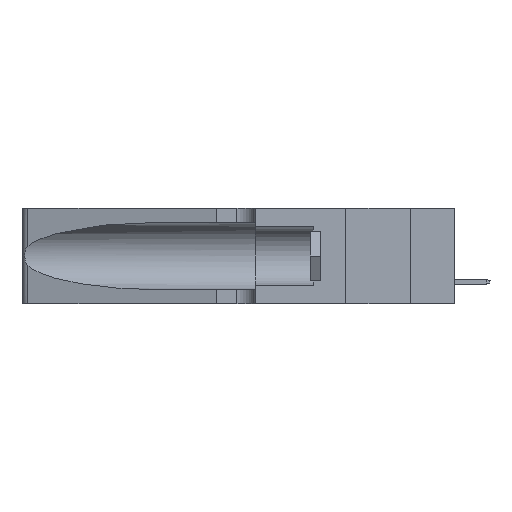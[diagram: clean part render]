
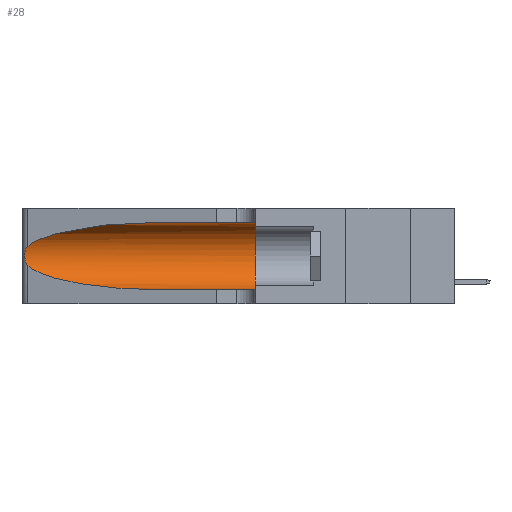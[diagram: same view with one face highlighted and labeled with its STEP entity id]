
A CAD part, left-side view. The second image highlights one B-rep face of the part: STEP entity #28.
In plain terms, the highlighted cylindrical face has radius 3.308 mm (diameter 6.617 mm), a partial arc.
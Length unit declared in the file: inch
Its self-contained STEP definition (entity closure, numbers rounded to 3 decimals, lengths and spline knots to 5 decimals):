
#28 = ADVANCED_FACE ( 'NONE', ( #6190 ), #16689, .F. ) ;
#848 = CARTESIAN_POINT ( 'NONE',  ( 0.25487, 1.22718, 0.14631 ) ) ;
#1458 = EDGE_CURVE ( 'NONE', #31231, #33976, #28889, .T. ) ;
#1917 = VERTEX_POINT ( 'NONE', #17736 ) ;
#2438 = CARTESIAN_POINT ( 'NONE',  ( 0.25487, 1.22718, 0.22369 ) ) ;
#2667 = EDGE_CURVE ( 'NONE', #25643, #31231, #16777, .T. ) ;
#3200 = ORIENTED_EDGE ( 'NONE', *, *, #5541, .F. ) ;
#3679 = CARTESIAN_POINT ( 'NONE',  ( 0.1305, 0.72297, 0.05475 ) ) ;
#3865 = CARTESIAN_POINT ( 'NONE',  ( 0.1305, 0.72297, 0.31525 ) ) ;
#3956 = DIRECTION ( 'NONE',  ( 0., 0., -1. ) ) ;
#4356 = CARTESIAN_POINT ( 'NONE',  ( 0.25487, 1.22718, 0.14631 ) ) ;
#4912 =( BOUNDED_CURVE ( )  B_SPLINE_CURVE ( 3, ( #9679, #20197, #30686, #3679 ),
 .UNSPECIFIED., .F., .T. ) 
 B_SPLINE_CURVE_WITH_KNOTS ( ( 4, 4 ),
 ( 3.44316, 4.71239 ),
 .UNSPECIFIED. ) 
 CURVE ( )  GEOMETRIC_REPRESENTATION_ITEM ( )  RATIONAL_B_SPLINE_CURVE ( ( 1., 0.87, 0.87, 1. ) ) 
 REPRESENTATION_ITEM ( '' )  );
#4992 = DIRECTION ( 'NONE',  ( 0., 1., 0. ) ) ;
#5541 = EDGE_CURVE ( 'NONE', #1917, #24523, #21792, .T. ) ;
#6121 = DIRECTION ( 'NONE',  ( 0., -1., 0. ) ) ;
#6190 = FACE_OUTER_BOUND ( 'NONE', #11603, .T. ) ;
#6216 = VERTEX_POINT ( 'NONE', #15237 ) ;
#6430 = CARTESIAN_POINT ( 'NONE',  ( 0.1305, 1.61858, 0.31525 ) ) ;
#6464 = CARTESIAN_POINT ( 'NONE',  ( 0.1305, 1.61858, 0.05475 ) ) ;
#6635 = EDGE_CURVE ( 'NONE', #33976, #6216, #4912, .T. ) ;
#6663 = EDGE_CURVE ( 'NONE', #25643, #1917, #30012, .T. ) ;
#7116 = ORIENTED_EDGE ( 'NONE', *, *, #6663, .F. ) ;
#7269 = CARTESIAN_POINT ( 'NONE',  ( 0.25639, 1.23186, 0.15144 ) ) ;
#7533 = AXIS2_PLACEMENT_3D ( 'NONE', #27198, #22193, #3956 ) ;
#7562 = VECTOR ( 'NONE', #32745, 39.37008 ) ;
#7593 = CARTESIAN_POINT ( 'NONE',  ( 0.25854, 1.2359, 0.20912 ) ) ;
#7616 = ORIENTED_EDGE ( 'NONE', *, *, #6635, .T. ) ;
#8374 = ORIENTED_EDGE ( 'NONE', *, *, #2667, .T. ) ;
#9072 = CARTESIAN_POINT ( 'NONE',  ( 0.1305, 0.35, 0.05475 ) ) ;
#9679 = CARTESIAN_POINT ( 'NONE',  ( 0.25487, 1.22718, 0.14631 ) ) ;
#10350 = CARTESIAN_POINT ( 'NONE',  ( 0.2373, 1.15595, 0.28018 ) ) ;
#11603 = EDGE_LOOP ( 'NONE', ( #8374, #33777, #7616, #32934, #3200, #7116 ) ) ;
#12437 = CARTESIAN_POINT ( 'NONE',  ( 0.26075, 1.23896, 0.178 ) ) ;
#12606 = CARTESIAN_POINT ( 'NONE',  ( 0.25639, 1.23184, 0.21858 ) ) ;
#15237 = CARTESIAN_POINT ( 'NONE',  ( 0.1305, 0.72297, 0.05475 ) ) ;
#15377 = EDGE_CURVE ( 'NONE', #6216, #24523, #24540, .T. ) ;
#16689 = CYLINDRICAL_SURFACE ( 'NONE', #7533, 0.13025 ) ;
#16777 =( BOUNDED_CURVE ( )  B_SPLINE_CURVE ( 3, ( #30860, #18119, #10350, #2438 ),
 .UNSPECIFIED., .F., .F. ) 
 B_SPLINE_CURVE_WITH_KNOTS ( ( 4, 4 ),
 ( 1.5708, 2.84003 ),
 .UNSPECIFIED. ) 
 CURVE ( )  GEOMETRIC_REPRESENTATION_ITEM ( )  RATIONAL_B_SPLINE_CURVE ( ( 1., 0.87, 0.87, 1. ) ) 
 REPRESENTATION_ITEM ( '' )  );
#17431 = CARTESIAN_POINT ( 'NONE',  ( 0.26017, 1.23833, 0.17102 ) ) ;
#17736 = CARTESIAN_POINT ( 'NONE',  ( 0.1305, 0.35, 0.31525 ) ) ;
#17781 = CARTESIAN_POINT ( 'NONE',  ( 0.26018, 1.23835, 0.19895 ) ) ;
#18116 = CARTESIAN_POINT ( 'NONE',  ( 0.26075, 1.23896, 0.19203 ) ) ;
#18119 = CARTESIAN_POINT ( 'NONE',  ( 0.18966, 0.96281, 0.31525 ) ) ;
#20197 = CARTESIAN_POINT ( 'NONE',  ( 0.2373, 1.15595, 0.08982 ) ) ;
#20545 = VECTOR ( 'NONE', #6121, 39.37008 ) ;
#20812 = DIRECTION ( 'NONE',  ( 0., 0., 1. ) ) ;
#21792 = CIRCLE ( 'NONE', #26768, 0.13025 ) ;
#22193 = DIRECTION ( 'NONE',  ( 0., -1., 0. ) ) ;
#22942 = CARTESIAN_POINT ( 'NONE',  ( 0.25789, 1.23486, 0.15765 ) ) ;
#23234 = CARTESIAN_POINT ( 'NONE',  ( 0.1305, 0.35, 0.185 ) ) ;
#24523 = VERTEX_POINT ( 'NONE', #9072 ) ;
#24540 = LINE ( 'NONE', #6464, #20545 ) ;
#25358 = CARTESIAN_POINT ( 'NONE',  ( 0.25555, 1.22993, 0.14849 ) ) ;
#25643 = VERTEX_POINT ( 'NONE', #3865 ) ;
#26768 = AXIS2_PLACEMENT_3D ( 'NONE', #23234, #4992, #20812 ) ;
#27198 = CARTESIAN_POINT ( 'NONE',  ( 0.1305, 1.61858, 0.185 ) ) ;
#27929 = CARTESIAN_POINT ( 'NONE',  ( 0.25856, 1.23593, 0.16098 ) ) ;
#28889 = B_SPLINE_CURVE_WITH_KNOTS ( 'NONE', 3,
 ( #31176, #30853, #12606, #30505, #7593, #17781, #18116, #12437, #17431, #27929, #22942, #7269, #25358, #4356 ),
 .UNSPECIFIED., .F., .F.,
 ( 4, 2, 2, 2, 2, 2, 4 ),
 ( 0., 0.00027, 0.00053, 0.00107, 0.0016, 0.00187, 0.00214 ),
 .UNSPECIFIED. ) ;
#30012 = LINE ( 'NONE', #6430, #7562 ) ;
#30505 = CARTESIAN_POINT ( 'NONE',  ( 0.25787, 1.23484, 0.2124 ) ) ;
#30686 = CARTESIAN_POINT ( 'NONE',  ( 0.18966, 0.96281, 0.05475 ) ) ;
#30853 = CARTESIAN_POINT ( 'NONE',  ( 0.25555, 1.22994, 0.2215 ) ) ;
#30860 = CARTESIAN_POINT ( 'NONE',  ( 0.1305, 0.72297, 0.31525 ) ) ;
#31176 = CARTESIAN_POINT ( 'NONE',  ( 0.25487, 1.22718, 0.22369 ) ) ;
#31231 = VERTEX_POINT ( 'NONE', #33106 ) ;
#32745 = DIRECTION ( 'NONE',  ( 0., -1., 0. ) ) ;
#32934 = ORIENTED_EDGE ( 'NONE', *, *, #15377, .T. ) ;
#33106 = CARTESIAN_POINT ( 'NONE',  ( 0.25487, 1.22718, 0.22369 ) ) ;
#33777 = ORIENTED_EDGE ( 'NONE', *, *, #1458, .T. ) ;
#33976 = VERTEX_POINT ( 'NONE', #848 ) ;
